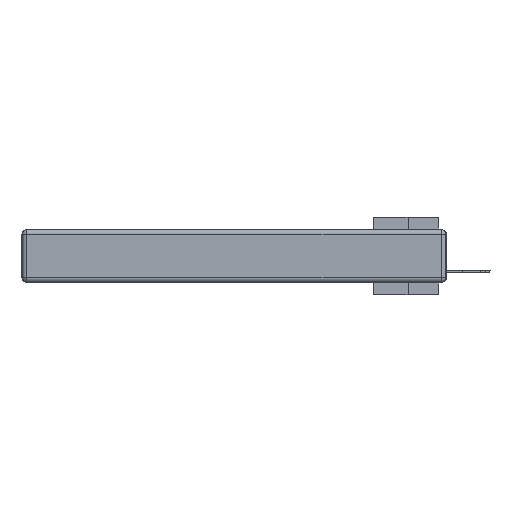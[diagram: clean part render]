
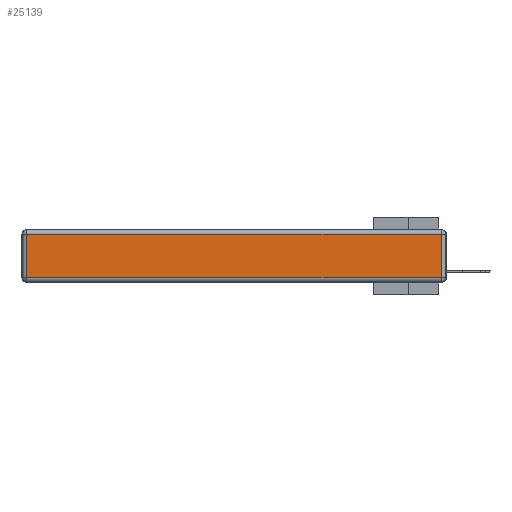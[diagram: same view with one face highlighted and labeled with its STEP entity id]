
A CAD part, left-side view. The second image highlights one B-rep face of the part: STEP entity #25139.
In plain terms, the highlighted planar face has unit normal (-1, 0, 0).
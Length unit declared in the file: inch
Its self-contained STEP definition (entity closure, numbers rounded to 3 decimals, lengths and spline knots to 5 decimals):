
#60 = ORIENTED_EDGE ( 'NONE', *, *, #28744, .T. ) ;
#381 = VECTOR ( 'NONE', #6932, 39.37008 ) ;
#2502 = FACE_OUTER_BOUND ( 'NONE', #26861, .T. ) ;
#4086 = ORIENTED_EDGE ( 'NONE', *, *, #32861, .T. ) ;
#4569 = VECTOR ( 'NONE', #11550, 39.37008 ) ;
#6932 = DIRECTION ( 'NONE',  ( 0., -1., 0. ) ) ;
#9053 = LINE ( 'NONE', #9940, #381 ) ;
#9216 = VECTOR ( 'NONE', #22166, 39.37008 ) ;
#9940 = CARTESIAN_POINT ( 'NONE',  ( 0., 0., -0.313 ) ) ;
#11076 = CARTESIAN_POINT ( 'NONE',  ( 0., 0.03, -0.03 ) ) ;
#11187 = PLANE ( 'NONE',  #23594 ) ;
#11550 = DIRECTION ( 'NONE',  ( 0., 0., 1. ) ) ;
#12636 = VECTOR ( 'NONE', #25955, 39.37008 ) ;
#12753 = LINE ( 'NONE', #28083, #4569 ) ;
#12793 = VERTEX_POINT ( 'NONE', #32624 ) ;
#13869 = VERTEX_POINT ( 'NONE', #11076 ) ;
#14969 = EDGE_CURVE ( 'NONE', #24678, #13869, #12753, .T. ) ;
#16530 = CARTESIAN_POINT ( 'NONE',  ( 0., 0., -0.343 ) ) ;
#16663 = ORIENTED_EDGE ( 'NONE', *, *, #24305, .T. ) ;
#18265 = LINE ( 'NONE', #23161, #12636 ) ;
#21402 = VERTEX_POINT ( 'NONE', #26275 ) ;
#22166 = DIRECTION ( 'NONE',  ( 0., 1., 0. ) ) ;
#22277 = CARTESIAN_POINT ( 'NONE',  ( 0., 2.75, -0.03 ) ) ;
#22546 = CARTESIAN_POINT ( 'NONE',  ( 0., 0.03, -0.313 ) ) ;
#23161 = CARTESIAN_POINT ( 'NONE',  ( 0., 2.72, -0.343 ) ) ;
#23594 = AXIS2_PLACEMENT_3D ( 'NONE', #16530, #33071, #25061 ) ;
#24305 = EDGE_CURVE ( 'NONE', #21402, #24678, #9053, .T. ) ;
#24678 = VERTEX_POINT ( 'NONE', #22546 ) ;
#25061 = DIRECTION ( 'NONE',  ( 0., 0., 1. ) ) ;
#25139 = ADVANCED_FACE ( 'NONE', ( #2502 ), #11187, .T. ) ;
#25719 = ORIENTED_EDGE ( 'NONE', *, *, #14969, .T. ) ;
#25955 = DIRECTION ( 'NONE',  ( 0., 0., -1. ) ) ;
#26275 = CARTESIAN_POINT ( 'NONE',  ( 0., 2.72, -0.313 ) ) ;
#26861 = EDGE_LOOP ( 'NONE', ( #16663, #25719, #60, #4086 ) ) ;
#28083 = CARTESIAN_POINT ( 'NONE',  ( 0., 0.03, -0.343 ) ) ;
#28744 = EDGE_CURVE ( 'NONE', #13869, #12793, #31234, .T. ) ;
#31234 = LINE ( 'NONE', #22277, #9216 ) ;
#32624 = CARTESIAN_POINT ( 'NONE',  ( 0., 2.72, -0.03 ) ) ;
#32861 = EDGE_CURVE ( 'NONE', #12793, #21402, #18265, .T. ) ;
#33071 = DIRECTION ( 'NONE',  ( -1., 0., 0. ) ) ;
